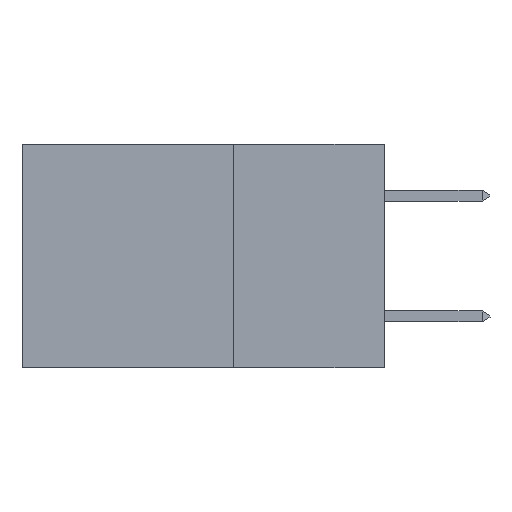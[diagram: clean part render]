
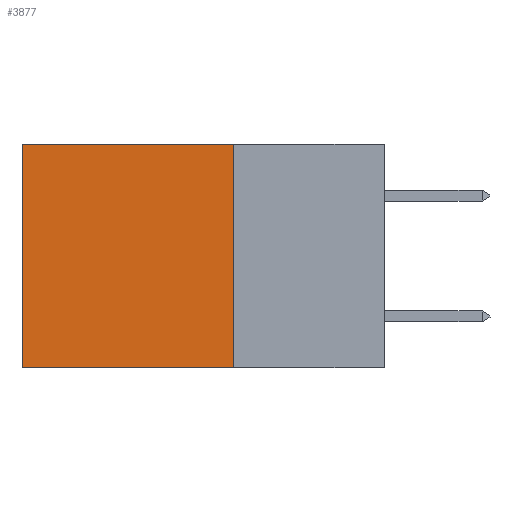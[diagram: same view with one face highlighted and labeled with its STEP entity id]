
A CAD part, left-side view. The second image highlights one B-rep face of the part: STEP entity #3877.
In plain terms, the highlighted planar face has unit normal (-1, 0, 0).
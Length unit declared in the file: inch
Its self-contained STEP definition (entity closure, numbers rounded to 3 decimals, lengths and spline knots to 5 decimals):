
#480 = LINE ( 'NONE', #15819, #8736 ) ;
#835 = CARTESIAN_POINT ( 'NONE',  ( 0.2875, 0.25, 0. ) ) ;
#1169 = LINE ( 'NONE', #16111, #16765 ) ;
#2407 = LINE ( 'NONE', #9910, #17985 ) ;
#2418 = DIRECTION ( 'NONE',  ( 1., 0., 0. ) ) ;
#3720 = DIRECTION ( 'NONE',  ( 0., 1., 0. ) ) ;
#3877 = ADVANCED_FACE ( 'NONE', ( #11965 ), #10141, .F. ) ;
#3881 = VERTEX_POINT ( 'NONE', #5514 ) ;
#4281 = EDGE_CURVE ( 'NONE', #18019, #3881, #480, .T. ) ;
#5399 = VERTEX_POINT ( 'NONE', #6761 ) ;
#5514 = CARTESIAN_POINT ( 'NONE',  ( 0.2875, 0.6, -0.37 ) ) ;
#5840 = EDGE_CURVE ( 'NONE', #8871, #3881, #17463, .T. ) ;
#6266 = CARTESIAN_POINT ( 'NONE',  ( 0.2875, 0.6, 0. ) ) ;
#6436 = DIRECTION ( 'NONE',  ( 0., 1., 0. ) ) ;
#6761 = CARTESIAN_POINT ( 'NONE',  ( 0.2875, 0.25, 0. ) ) ;
#7304 = CARTESIAN_POINT ( 'NONE',  ( 0.2875, 0.6, 0. ) ) ;
#7858 = DIRECTION ( 'NONE',  ( 0., 0., -1. ) ) ;
#7877 = EDGE_CURVE ( 'NONE', #5399, #8871, #1169, .T. ) ;
#7991 = EDGE_CURVE ( 'NONE', #5399, #18019, #2407, .T. ) ;
#8223 = AXIS2_PLACEMENT_3D ( 'NONE', #835, #2418, #13309 ) ;
#8355 = DIRECTION ( 'NONE',  ( 0., 0., -1. ) ) ;
#8736 = VECTOR ( 'NONE', #6436, 39.37008 ) ;
#8871 = VERTEX_POINT ( 'NONE', #7304 ) ;
#9910 = CARTESIAN_POINT ( 'NONE',  ( 0.2875, 0.25, 0. ) ) ;
#10141 = PLANE ( 'NONE',  #8223 ) ;
#11723 = EDGE_LOOP ( 'NONE', ( #14819, #13442, #16596, #17734 ) ) ;
#11965 = FACE_OUTER_BOUND ( 'NONE', #11723, .T. ) ;
#13309 = DIRECTION ( 'NONE',  ( 0., 0., -1. ) ) ;
#13314 = CARTESIAN_POINT ( 'NONE',  ( 0.2875, 0.25, -0.37 ) ) ;
#13442 = ORIENTED_EDGE ( 'NONE', *, *, #4281, .F. ) ;
#14819 = ORIENTED_EDGE ( 'NONE', *, *, #5840, .T. ) ;
#15819 = CARTESIAN_POINT ( 'NONE',  ( 0.2875, 0.25, -0.37 ) ) ;
#16111 = CARTESIAN_POINT ( 'NONE',  ( 0.2875, 0.25, 0. ) ) ;
#16596 = ORIENTED_EDGE ( 'NONE', *, *, #7991, .F. ) ;
#16765 = VECTOR ( 'NONE', #3720, 39.37008 ) ;
#17463 = LINE ( 'NONE', #6266, #18433 ) ;
#17734 = ORIENTED_EDGE ( 'NONE', *, *, #7877, .T. ) ;
#17985 = VECTOR ( 'NONE', #8355, 39.37008 ) ;
#18019 = VERTEX_POINT ( 'NONE', #13314 ) ;
#18433 = VECTOR ( 'NONE', #7858, 39.37008 ) ;
